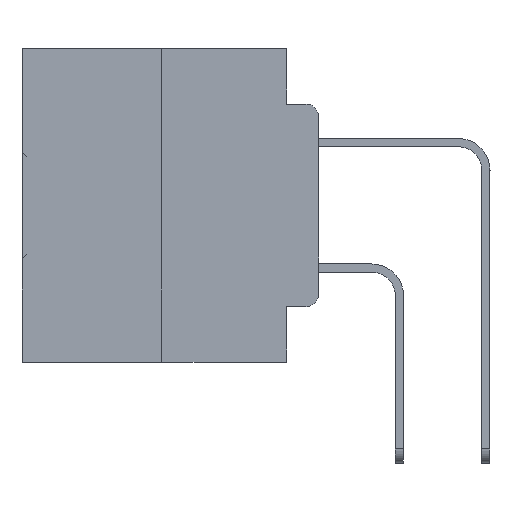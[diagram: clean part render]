
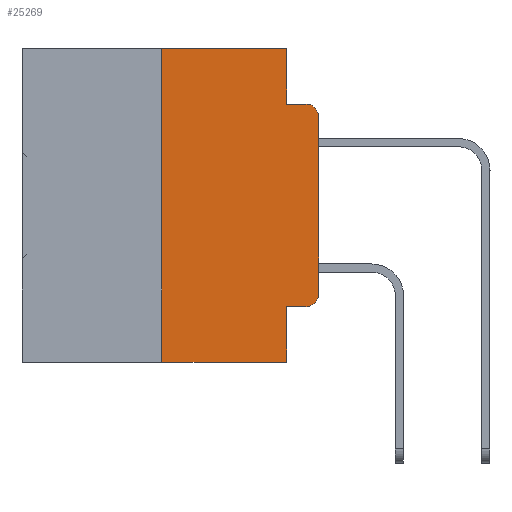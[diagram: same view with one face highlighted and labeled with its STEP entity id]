
A CAD part, left-side view. The second image highlights one B-rep face of the part: STEP entity #25269.
In plain terms, the highlighted planar face has unit normal (-1, 0, 0).
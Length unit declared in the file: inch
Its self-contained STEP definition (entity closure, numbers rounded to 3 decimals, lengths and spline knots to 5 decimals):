
#1145 = VERTEX_POINT ( 'NONE', #10808 ) ;
#1223 = DIRECTION ( 'NONE',  ( 1., 0., 0. ) ) ;
#1405 = CARTESIAN_POINT ( 'NONE',  ( 0., 0.02, -0.3915 ) ) ;
#2086 = VERTEX_POINT ( 'NONE', #15118 ) ;
#2687 = DIRECTION ( 'NONE',  ( 0., -1., 0. ) ) ;
#3053 = VECTOR ( 'NONE', #34015, 39.37008 ) ;
#3324 = AXIS2_PLACEMENT_3D ( 'NONE', #1405, #6875, #18098 ) ;
#3450 = ORIENTED_EDGE ( 'NONE', *, *, #4203, .T. ) ;
#4042 = VECTOR ( 'NONE', #31792, 39.37008 ) ;
#4203 = EDGE_CURVE ( 'NONE', #26699, #1145, #19036, .T. ) ;
#4290 = FACE_OUTER_BOUND ( 'NONE', #15883, .T. ) ;
#4323 = CARTESIAN_POINT ( 'NONE',  ( 0., 0.02, -0.4115 ) ) ;
#4417 = LINE ( 'NONE', #22499, #13813 ) ;
#4796 = CARTESIAN_POINT ( 'NONE',  ( 0., 0.473, -0.5 ) ) ;
#5621 = EDGE_CURVE ( 'NONE', #5714, #34207, #23802, .T. ) ;
#5714 = VERTEX_POINT ( 'NONE', #16867 ) ;
#6113 = CARTESIAN_POINT ( 'NONE',  ( 0., 0.051, 0. ) ) ;
#6875 = DIRECTION ( 'NONE',  ( -1., 0., 0. ) ) ;
#7048 = DIRECTION ( 'NONE',  ( -1., 0., 0. ) ) ;
#7127 = VERTEX_POINT ( 'NONE', #4323 ) ;
#7182 = DIRECTION ( 'NONE',  ( 0., 0., -1. ) ) ;
#9618 = CARTESIAN_POINT ( 'NONE',  ( 0., 0.25, 0. ) ) ;
#9703 = CARTESIAN_POINT ( 'NONE',  ( 0., 0.051, -0.5 ) ) ;
#10652 = LINE ( 'NONE', #28269, #3053 ) ;
#10808 = CARTESIAN_POINT ( 'NONE',  ( 0., 0.02, -0.0885 ) ) ;
#11173 = ORIENTED_EDGE ( 'NONE', *, *, #19758, .F. ) ;
#11822 = AXIS2_PLACEMENT_3D ( 'NONE', #15579, #7048, #7182 ) ;
#12646 = EDGE_CURVE ( 'NONE', #2086, #34207, #4417, .T. ) ;
#13015 = EDGE_CURVE ( 'NONE', #15167, #26699, #10652, .T. ) ;
#13115 = PLANE ( 'NONE',  #21136 ) ;
#13378 = ORIENTED_EDGE ( 'NONE', *, *, #19320, .T. ) ;
#13443 = DIRECTION ( 'NONE',  ( 0., -1., 0. ) ) ;
#13813 = VECTOR ( 'NONE', #31251, 39.37008 ) ;
#13961 = ORIENTED_EDGE ( 'NONE', *, *, #32651, .F. ) ;
#15118 = CARTESIAN_POINT ( 'NONE',  ( 0., 0.051, -0.4115 ) ) ;
#15167 = VERTEX_POINT ( 'NONE', #18576 ) ;
#15579 = CARTESIAN_POINT ( 'NONE',  ( 0., 0.02, -0.1085 ) ) ;
#15883 = EDGE_LOOP ( 'NONE', ( #23885, #3450, #28062, #11173, #32033, #13961, #36428, #27521, #27319, #13378 ) ) ;
#16279 = VECTOR ( 'NONE', #13443, 39.37008 ) ;
#16283 = VECTOR ( 'NONE', #16575, 39.37008 ) ;
#16575 = DIRECTION ( 'NONE',  ( 0., 0., 1. ) ) ;
#16588 = EDGE_CURVE ( 'NONE', #2086, #7127, #36713, .T. ) ;
#16867 = CARTESIAN_POINT ( 'NONE',  ( 0., 0.25, -0.5 ) ) ;
#18098 = DIRECTION ( 'NONE',  ( 0., 0., -1. ) ) ;
#18305 = CARTESIAN_POINT ( 'NONE',  ( 0., 0.051, -0.0885 ) ) ;
#18431 = VECTOR ( 'NONE', #2687, 39.37008 ) ;
#18576 = CARTESIAN_POINT ( 'NONE',  ( 0., 0., -0.3915 ) ) ;
#18614 = LINE ( 'NONE', #18305, #31974 ) ;
#19036 = CIRCLE ( 'NONE', #11822, 0.02 ) ;
#19320 = EDGE_CURVE ( 'NONE', #7127, #15167, #24148, .T. ) ;
#19405 = VECTOR ( 'NONE', #33095, 39.37008 ) ;
#19427 = CARTESIAN_POINT ( 'NONE',  ( 0., 0.051, 0. ) ) ;
#19758 = EDGE_CURVE ( 'NONE', #33833, #29546, #33079, .T. ) ;
#21136 = AXIS2_PLACEMENT_3D ( 'NONE', #27286, #1223, #33021 ) ;
#22499 = CARTESIAN_POINT ( 'NONE',  ( 0., 0.051, 0. ) ) ;
#22803 = CARTESIAN_POINT ( 'NONE',  ( 0., 0.051, -0.0885 ) ) ;
#23802 = LINE ( 'NONE', #4796, #16279 ) ;
#23805 = LINE ( 'NONE', #25013, #16283 ) ;
#23885 = ORIENTED_EDGE ( 'NONE', *, *, #13015, .T. ) ;
#24148 = CIRCLE ( 'NONE', #3324, 0.02 ) ;
#24613 = VERTEX_POINT ( 'NONE', #9618 ) ;
#24801 = EDGE_CURVE ( 'NONE', #29546, #1145, #18614, .T. ) ;
#25013 = CARTESIAN_POINT ( 'NONE',  ( 0., 0.25, 0. ) ) ;
#25269 = ADVANCED_FACE ( 'NONE', ( #4290 ), #13115, .F. ) ;
#26699 = VERTEX_POINT ( 'NONE', #36110 ) ;
#27229 = CARTESIAN_POINT ( 'NONE',  ( 0., 0.473, 0. ) ) ;
#27286 = CARTESIAN_POINT ( 'NONE',  ( 0., 0.473, 0. ) ) ;
#27319 = ORIENTED_EDGE ( 'NONE', *, *, #16588, .T. ) ;
#27521 = ORIENTED_EDGE ( 'NONE', *, *, #12646, .F. ) ;
#28062 = ORIENTED_EDGE ( 'NONE', *, *, #24801, .F. ) ;
#28269 = CARTESIAN_POINT ( 'NONE',  ( 0., 0., 0. ) ) ;
#29546 = VERTEX_POINT ( 'NONE', #22803 ) ;
#30655 = CARTESIAN_POINT ( 'NONE',  ( 0., 0.051, -0.4115 ) ) ;
#31251 = DIRECTION ( 'NONE',  ( 0., 0., -1. ) ) ;
#31480 = LINE ( 'NONE', #27229, #19405 ) ;
#31792 = DIRECTION ( 'NONE',  ( 0., 0., -1. ) ) ;
#31974 = VECTOR ( 'NONE', #33669, 39.37008 ) ;
#32033 = ORIENTED_EDGE ( 'NONE', *, *, #36412, .F. ) ;
#32651 = EDGE_CURVE ( 'NONE', #5714, #24613, #23805, .T. ) ;
#33021 = DIRECTION ( 'NONE',  ( 0., 0., -1. ) ) ;
#33079 = LINE ( 'NONE', #6113, #4042 ) ;
#33095 = DIRECTION ( 'NONE',  ( 0., -1., 0. ) ) ;
#33669 = DIRECTION ( 'NONE',  ( 0., -1., 0. ) ) ;
#33833 = VERTEX_POINT ( 'NONE', #19427 ) ;
#34015 = DIRECTION ( 'NONE',  ( 0., 0., 1. ) ) ;
#34207 = VERTEX_POINT ( 'NONE', #9703 ) ;
#36110 = CARTESIAN_POINT ( 'NONE',  ( 0., 0., -0.1085 ) ) ;
#36412 = EDGE_CURVE ( 'NONE', #24613, #33833, #31480, .T. ) ;
#36428 = ORIENTED_EDGE ( 'NONE', *, *, #5621, .T. ) ;
#36713 = LINE ( 'NONE', #30655, #18431 ) ;
